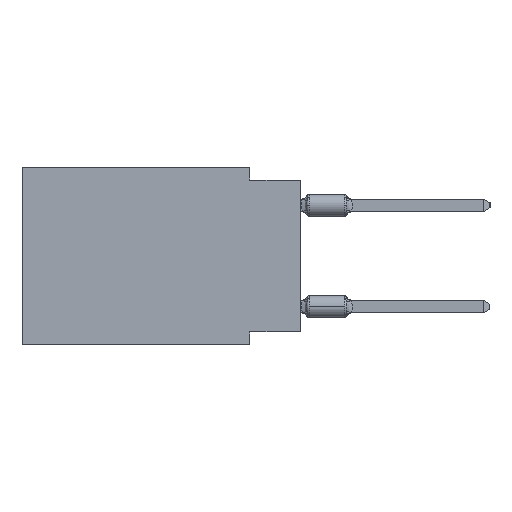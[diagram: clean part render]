
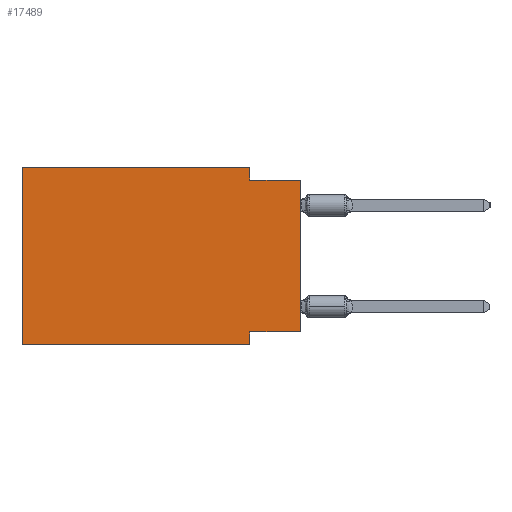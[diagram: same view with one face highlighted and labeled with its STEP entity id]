
A CAD part, left-side view. The second image highlights one B-rep face of the part: STEP entity #17489.
In plain terms, the highlighted planar face has unit normal (-1, 0, 0).
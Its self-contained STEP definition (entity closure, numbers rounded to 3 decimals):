
#564 = CARTESIAN_POINT ( 'NONE',  ( 0., 0., -8.255 ) ) ;
#1411 = CARTESIAN_POINT ( 'NONE',  ( 0., 13.97, 0. ) ) ;
#1717 = EDGE_CURVE ( 'NONE', #21830, #32916, #3747, .T. ) ;
#1799 = VECTOR ( 'NONE', #20144, 1000. ) ;
#2519 = EDGE_CURVE ( 'NONE', #21830, #7622, #7999, .T. ) ;
#2774 = CARTESIAN_POINT ( 'NONE',  ( 0., 0., -0.635 ) ) ;
#3747 = LINE ( 'NONE', #564, #24938 ) ;
#3793 = CARTESIAN_POINT ( 'NONE',  ( 0., 13.97, -8.89 ) ) ;
#3822 = ORIENTED_EDGE ( 'NONE', *, *, #30723, .F. ) ;
#4929 = VECTOR ( 'NONE', #28521, 1000. ) ;
#5053 = ORIENTED_EDGE ( 'NONE', *, *, #23875, .F. ) ;
#5876 = CARTESIAN_POINT ( 'NONE',  ( 0., 13.97, -8.89 ) ) ;
#6073 = LINE ( 'NONE', #17212, #4929 ) ;
#6078 = EDGE_CURVE ( 'NONE', #32916, #25808, #17964, .T. ) ;
#7622 = VERTEX_POINT ( 'NONE', #28563 ) ;
#7999 = LINE ( 'NONE', #19529, #37043 ) ;
#8503 = VERTEX_POINT ( 'NONE', #23409 ) ;
#8937 = VECTOR ( 'NONE', #10883, 1000. ) ;
#9014 = EDGE_CURVE ( 'NONE', #13044, #7622, #19958, .T. ) ;
#10883 = DIRECTION ( 'NONE',  ( 0., 0., 1. ) ) ;
#10890 = LINE ( 'NONE', #25241, #11081 ) ;
#11081 = VECTOR ( 'NONE', #22423, 1000. ) ;
#11198 = ORIENTED_EDGE ( 'NONE', *, *, #2519, .T. ) ;
#13044 = VERTEX_POINT ( 'NONE', #16224 ) ;
#14881 = ORIENTED_EDGE ( 'NONE', *, *, #9014, .F. ) ;
#15700 = ORIENTED_EDGE ( 'NONE', *, *, #20540, .F. ) ;
#16224 = CARTESIAN_POINT ( 'NONE',  ( 0., 2.54, -0.635 ) ) ;
#16415 = CARTESIAN_POINT ( 'NONE',  ( 0., 13.97, 0. ) ) ;
#17212 = CARTESIAN_POINT ( 'NONE',  ( 0., 2.54, 0. ) ) ;
#17489 = ADVANCED_FACE ( 'NONE', ( #21428 ), #35736, .F. ) ;
#17964 = LINE ( 'NONE', #21357, #29346 ) ;
#18147 = LINE ( 'NONE', #3793, #25212 ) ;
#19529 = CARTESIAN_POINT ( 'NONE',  ( 0., 0., 0. ) ) ;
#19958 = LINE ( 'NONE', #2774, #1799 ) ;
#20144 = DIRECTION ( 'NONE',  ( 0., -1., 0. ) ) ;
#20243 = CARTESIAN_POINT ( 'NONE',  ( 0., 2.54, -8.255 ) ) ;
#20540 = EDGE_CURVE ( 'NONE', #8503, #13044, #6073, .T. ) ;
#20742 = EDGE_CURVE ( 'NONE', #23629, #25808, #18147, .T. ) ;
#21357 = CARTESIAN_POINT ( 'NONE',  ( 0., 2.54, -8.89 ) ) ;
#21428 = FACE_OUTER_BOUND ( 'NONE', #35676, .T. ) ;
#21830 = VERTEX_POINT ( 'NONE', #33286 ) ;
#22423 = DIRECTION ( 'NONE',  ( 0., -1., 0. ) ) ;
#23409 = CARTESIAN_POINT ( 'NONE',  ( 0., 2.54, 0. ) ) ;
#23629 = VERTEX_POINT ( 'NONE', #5876 ) ;
#23875 = EDGE_CURVE ( 'NONE', #30268, #8503, #10890, .T. ) ;
#24083 = DIRECTION ( 'NONE',  ( 1., 0., 0. ) ) ;
#24295 = ORIENTED_EDGE ( 'NONE', *, *, #20742, .T. ) ;
#24938 = VECTOR ( 'NONE', #29785, 1000. ) ;
#25212 = VECTOR ( 'NONE', #35668, 1000. ) ;
#25241 = CARTESIAN_POINT ( 'NONE',  ( 0., 13.97, 0. ) ) ;
#25808 = VERTEX_POINT ( 'NONE', #31679 ) ;
#26654 = ORIENTED_EDGE ( 'NONE', *, *, #6078, .F. ) ;
#28521 = DIRECTION ( 'NONE',  ( 0., 0., -1. ) ) ;
#28563 = CARTESIAN_POINT ( 'NONE',  ( 0., 0., -0.635 ) ) ;
#28714 = DIRECTION ( 'NONE',  ( 0., 0., 1. ) ) ;
#29346 = VECTOR ( 'NONE', #29469, 1000. ) ;
#29469 = DIRECTION ( 'NONE',  ( 0., 0., -1. ) ) ;
#29785 = DIRECTION ( 'NONE',  ( 0., 1., 0. ) ) ;
#30268 = VERTEX_POINT ( 'NONE', #16415 ) ;
#30723 = EDGE_CURVE ( 'NONE', #23629, #30268, #34453, .T. ) ;
#31324 = AXIS2_PLACEMENT_3D ( 'NONE', #1411, #24083, #35555 ) ;
#31679 = CARTESIAN_POINT ( 'NONE',  ( 0., 2.54, -8.89 ) ) ;
#32916 = VERTEX_POINT ( 'NONE', #20243 ) ;
#33078 = ORIENTED_EDGE ( 'NONE', *, *, #1717, .F. ) ;
#33286 = CARTESIAN_POINT ( 'NONE',  ( 0., 0., -8.255 ) ) ;
#33880 = CARTESIAN_POINT ( 'NONE',  ( 0., 13.97, 0. ) ) ;
#34453 = LINE ( 'NONE', #33880, #8937 ) ;
#35555 = DIRECTION ( 'NONE',  ( 0., 0., -1. ) ) ;
#35668 = DIRECTION ( 'NONE',  ( 0., -1., 0. ) ) ;
#35676 = EDGE_LOOP ( 'NONE', ( #11198, #14881, #15700, #5053, #3822, #24295, #26654, #33078 ) ) ;
#35736 = PLANE ( 'NONE',  #31324 ) ;
#37043 = VECTOR ( 'NONE', #28714, 1000. ) ;
